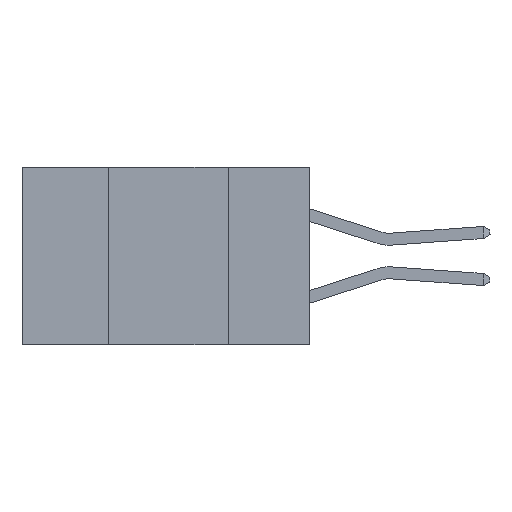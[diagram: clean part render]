
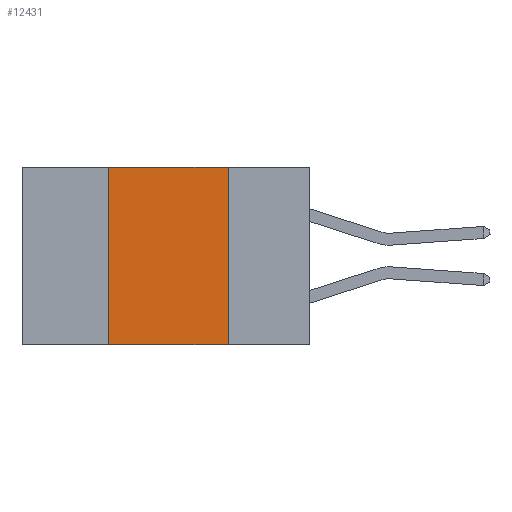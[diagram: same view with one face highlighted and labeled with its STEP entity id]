
A CAD part, left-side view. The second image highlights one B-rep face of the part: STEP entity #12431.
In plain terms, the highlighted planar face has unit normal (-1, 0, 0).
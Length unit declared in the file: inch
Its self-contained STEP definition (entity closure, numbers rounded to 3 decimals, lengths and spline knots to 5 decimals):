
#80 = DIRECTION ( 'NONE',  ( 1., 0., 0. ) ) ;
#1231 = LINE ( 'NONE', #4253, #12566 ) ;
#1710 = CARTESIAN_POINT ( 'NONE',  ( 0., 0.6, 0. ) ) ;
#2293 = VERTEX_POINT ( 'NONE', #10694 ) ;
#3102 = VERTEX_POINT ( 'NONE', #5917 ) ;
#3608 = CARTESIAN_POINT ( 'NONE',  ( 0., 0.6, 0. ) ) ;
#4141 = DIRECTION ( 'NONE',  ( 0., -1., 0. ) ) ;
#4235 = CARTESIAN_POINT ( 'NONE',  ( 0., 0.42, 0. ) ) ;
#4253 = CARTESIAN_POINT ( 'NONE',  ( 0., 0.6, -0.37 ) ) ;
#4823 = PLANE ( 'NONE',  #11178 ) ;
#5032 = ORIENTED_EDGE ( 'NONE', *, *, #6168, .F. ) ;
#5093 = ORIENTED_EDGE ( 'NONE', *, *, #10572, .T. ) ;
#5704 = EDGE_CURVE ( 'NONE', #3102, #5748, #14536, .T. ) ;
#5748 = VERTEX_POINT ( 'NONE', #12093 ) ;
#5917 = CARTESIAN_POINT ( 'NONE',  ( 0., 0.17, 0. ) ) ;
#5968 = DIRECTION ( 'NONE',  ( 0., 0., 1. ) ) ;
#6168 = EDGE_CURVE ( 'NONE', #2293, #11575, #7875, .T. ) ;
#6206 = CARTESIAN_POINT ( 'NONE',  ( 0., 0.42, -0.37 ) ) ;
#6340 = ORIENTED_EDGE ( 'NONE', *, *, #5704, .F. ) ;
#6904 = CARTESIAN_POINT ( 'NONE',  ( 0., 0.17, -0.37 ) ) ;
#7346 = ORIENTED_EDGE ( 'NONE', *, *, #14497, .F. ) ;
#7875 = LINE ( 'NONE', #6206, #10398 ) ;
#8324 = DIRECTION ( 'NONE',  ( 0., 0., -1. ) ) ;
#8389 = VECTOR ( 'NONE', #8742, 39.37008 ) ;
#8742 = DIRECTION ( 'NONE',  ( 0., -1., 0. ) ) ;
#8898 = VECTOR ( 'NONE', #13776, 39.37008 ) ;
#10398 = VECTOR ( 'NONE', #5968, 39.37008 ) ;
#10562 = EDGE_LOOP ( 'NONE', ( #6340, #7346, #5032, #5093 ) ) ;
#10572 = EDGE_CURVE ( 'NONE', #2293, #5748, #1231, .T. ) ;
#10694 = CARTESIAN_POINT ( 'NONE',  ( 0., 0.42, -0.37 ) ) ;
#11178 = AXIS2_PLACEMENT_3D ( 'NONE', #3608, #80, #8324 ) ;
#11572 = LINE ( 'NONE', #1710, #8389 ) ;
#11575 = VERTEX_POINT ( 'NONE', #4235 ) ;
#12093 = CARTESIAN_POINT ( 'NONE',  ( 0., 0.17, -0.37 ) ) ;
#12431 = ADVANCED_FACE ( 'NONE', ( #14315 ), #4823, .F. ) ;
#12566 = VECTOR ( 'NONE', #4141, 39.37008 ) ;
#13776 = DIRECTION ( 'NONE',  ( 0., 0., -1. ) ) ;
#14315 = FACE_OUTER_BOUND ( 'NONE', #10562, .T. ) ;
#14497 = EDGE_CURVE ( 'NONE', #11575, #3102, #11572, .T. ) ;
#14536 = LINE ( 'NONE', #6904, #8898 ) ;
